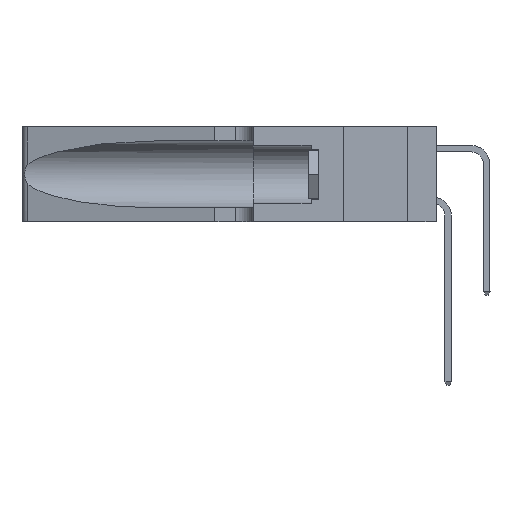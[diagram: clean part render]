
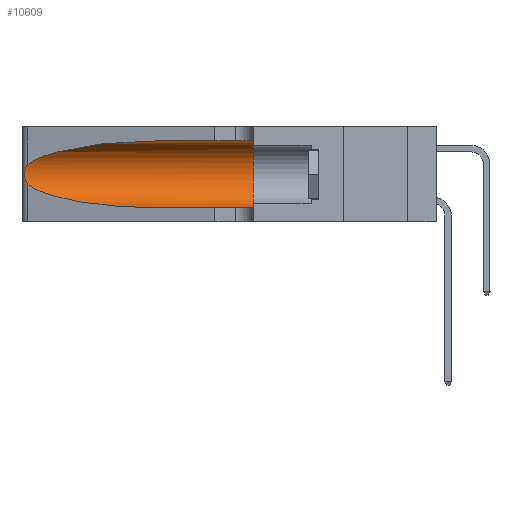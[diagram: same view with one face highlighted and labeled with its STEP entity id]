
A CAD part, left-side view. The second image highlights one B-rep face of the part: STEP entity #10609.
In plain terms, the highlighted cylindrical face has radius 3.308 mm (diameter 6.617 mm), a partial arc.
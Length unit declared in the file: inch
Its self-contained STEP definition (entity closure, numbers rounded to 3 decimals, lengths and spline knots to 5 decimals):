
#232 = CARTESIAN_POINT ( 'NONE',  ( 0.25789, 1.23486, 0.15765 ) ) ;
#282 = CARTESIAN_POINT ( 'NONE',  ( 0.25487, 1.22718, 0.22369 ) ) ;
#656 =( BOUNDED_CURVE ( )  B_SPLINE_CURVE ( 3, ( #3822, #26738, #10141, #18543 ),
 .UNSPECIFIED., .F., .F. ) 
 B_SPLINE_CURVE_WITH_KNOTS ( ( 4, 4 ),
 ( 3.44316, 4.71239 ),
 .UNSPECIFIED. ) 
 CURVE ( )  GEOMETRIC_REPRESENTATION_ITEM ( )  RATIONAL_B_SPLINE_CURVE ( ( 1., 0.87, 0.87, 1. ) ) 
 REPRESENTATION_ITEM ( '' )  );
#1777 = VERTEX_POINT ( 'NONE', #18138 ) ;
#2308 = CARTESIAN_POINT ( 'NONE',  ( 0.25487, 1.22718, 0.22369 ) ) ;
#2403 = CARTESIAN_POINT ( 'NONE',  ( 0.25555, 1.22993, 0.14849 ) ) ;
#2405 = ORIENTED_EDGE ( 'NONE', *, *, #3024, .F. ) ;
#3024 = EDGE_CURVE ( 'NONE', #24412, #22447, #14828, .T. ) ;
#3822 = CARTESIAN_POINT ( 'NONE',  ( 0.25487, 1.22718, 0.14631 ) ) ;
#3905 = EDGE_CURVE ( 'NONE', #4734, #1777, #20931, .T. ) ;
#4068 = EDGE_CURVE ( 'NONE', #20470, #4734, #656, .T. ) ;
#4179 = DIRECTION ( 'NONE',  ( 0., 1., 0. ) ) ;
#4346 = EDGE_LOOP ( 'NONE', ( #7255, #17045, #26488, #23386, #22606, #2405 ) ) ;
#4648 = DIRECTION ( 'NONE',  ( 0., -1., 0. ) ) ;
#4654 = CARTESIAN_POINT ( 'NONE',  ( 0.1305, 0.72297, 0.31525 ) ) ;
#4734 = VERTEX_POINT ( 'NONE', #20768 ) ;
#6615 = CARTESIAN_POINT ( 'NONE',  ( 0.25787, 1.23484, 0.2124 ) ) ;
#7255 = ORIENTED_EDGE ( 'NONE', *, *, #11817, .T. ) ;
#7945 = EDGE_CURVE ( 'NONE', #22447, #1777, #19527, .T. ) ;
#8757 = CARTESIAN_POINT ( 'NONE',  ( 0.26018, 1.23835, 0.19895 ) ) ;
#9828 = VECTOR ( 'NONE', #16001, 39.37008 ) ;
#10141 = CARTESIAN_POINT ( 'NONE',  ( 0.18966, 0.96281, 0.05475 ) ) ;
#10609 = ADVANCED_FACE ( 'NONE', ( #25759 ), #14796, .F. ) ;
#10856 = CARTESIAN_POINT ( 'NONE',  ( 0.26075, 1.23896, 0.178 ) ) ;
#11059 = DIRECTION ( 'NONE',  ( 0., 0., -1. ) ) ;
#11817 = EDGE_CURVE ( 'NONE', #24412, #23357, #25556, .T. ) ;
#11956 = CARTESIAN_POINT ( 'NONE',  ( 0.25487, 1.22718, 0.22369 ) ) ;
#12934 = CARTESIAN_POINT ( 'NONE',  ( 0.18966, 0.96281, 0.31525 ) ) ;
#12967 = CARTESIAN_POINT ( 'NONE',  ( 0.25856, 1.23593, 0.16098 ) ) ;
#13262 = CARTESIAN_POINT ( 'NONE',  ( 0.1305, 0.35, 0.31525 ) ) ;
#13805 = DIRECTION ( 'NONE',  ( 0., -1., 0. ) ) ;
#13936 = B_SPLINE_CURVE_WITH_KNOTS ( 'NONE', 3,
 ( #2308, #15007, #19188, #6615, #21249, #8757, #23313, #10856, #25390, #12967, #232, #15100, #2403, #17183 ),
 .UNSPECIFIED., .F., .F.,
 ( 4, 2, 2, 2, 2, 2, 4 ),
 ( 0., 0.00027, 0.00053, 0.00107, 0.0016, 0.00187, 0.00214 ),
 .UNSPECIFIED. ) ;
#14796 = CYLINDRICAL_SURFACE ( 'NONE', #25042, 0.13025 ) ;
#14828 = LINE ( 'NONE', #18005, #25161 ) ;
#15007 = CARTESIAN_POINT ( 'NONE',  ( 0.25555, 1.22994, 0.2215 ) ) ;
#15100 = CARTESIAN_POINT ( 'NONE',  ( 0.25639, 1.23186, 0.15144 ) ) ;
#16001 = DIRECTION ( 'NONE',  ( 0., -1., 0. ) ) ;
#16808 = CARTESIAN_POINT ( 'NONE',  ( 0.1305, 0.35, 0.185 ) ) ;
#16852 = CARTESIAN_POINT ( 'NONE',  ( 0.25487, 1.22718, 0.14631 ) ) ;
#17045 = ORIENTED_EDGE ( 'NONE', *, *, #22992, .T. ) ;
#17183 = CARTESIAN_POINT ( 'NONE',  ( 0.25487, 1.22718, 0.14631 ) ) ;
#18005 = CARTESIAN_POINT ( 'NONE',  ( 0.1305, 1.61858, 0.31525 ) ) ;
#18138 = CARTESIAN_POINT ( 'NONE',  ( 0.1305, 0.35, 0.05475 ) ) ;
#18355 = AXIS2_PLACEMENT_3D ( 'NONE', #16808, #4179, #18892 ) ;
#18543 = CARTESIAN_POINT ( 'NONE',  ( 0.1305, 0.72297, 0.05475 ) ) ;
#18892 = DIRECTION ( 'NONE',  ( 0., 0., 1. ) ) ;
#19188 = CARTESIAN_POINT ( 'NONE',  ( 0.25639, 1.23184, 0.21858 ) ) ;
#19527 = CIRCLE ( 'NONE', #18355, 0.13025 ) ;
#20470 = VERTEX_POINT ( 'NONE', #16852 ) ;
#20768 = CARTESIAN_POINT ( 'NONE',  ( 0.1305, 0.72297, 0.05475 ) ) ;
#20931 = LINE ( 'NONE', #22038, #9828 ) ;
#21249 = CARTESIAN_POINT ( 'NONE',  ( 0.25854, 1.2359, 0.20912 ) ) ;
#21300 = CARTESIAN_POINT ( 'NONE',  ( 0.2373, 1.15595, 0.28018 ) ) ;
#22038 = CARTESIAN_POINT ( 'NONE',  ( 0.1305, 1.61858, 0.05475 ) ) ;
#22447 = VERTEX_POINT ( 'NONE', #13262 ) ;
#22606 = ORIENTED_EDGE ( 'NONE', *, *, #7945, .F. ) ;
#22992 = EDGE_CURVE ( 'NONE', #23357, #20470, #13936, .T. ) ;
#23313 = CARTESIAN_POINT ( 'NONE',  ( 0.26075, 1.23896, 0.19203 ) ) ;
#23357 = VERTEX_POINT ( 'NONE', #11956 ) ;
#23386 = ORIENTED_EDGE ( 'NONE', *, *, #3905, .T. ) ;
#23514 = CARTESIAN_POINT ( 'NONE',  ( 0.1305, 1.61858, 0.185 ) ) ;
#24412 = VERTEX_POINT ( 'NONE', #4654 ) ;
#25042 = AXIS2_PLACEMENT_3D ( 'NONE', #23514, #4648, #11059 ) ;
#25161 = VECTOR ( 'NONE', #13805, 39.37008 ) ;
#25390 = CARTESIAN_POINT ( 'NONE',  ( 0.26017, 1.23833, 0.17102 ) ) ;
#25449 = CARTESIAN_POINT ( 'NONE',  ( 0.1305, 0.72297, 0.31525 ) ) ;
#25556 =( BOUNDED_CURVE ( )  B_SPLINE_CURVE ( 3, ( #25449, #12934, #21300, #282 ),
 .UNSPECIFIED., .F., .F. ) 
 B_SPLINE_CURVE_WITH_KNOTS ( ( 4, 4 ),
 ( 1.5708, 2.84003 ),
 .UNSPECIFIED. ) 
 CURVE ( )  GEOMETRIC_REPRESENTATION_ITEM ( )  RATIONAL_B_SPLINE_CURVE ( ( 1., 0.87, 0.87, 1. ) ) 
 REPRESENTATION_ITEM ( '' )  );
#25759 = FACE_OUTER_BOUND ( 'NONE', #4346, .T. ) ;
#26488 = ORIENTED_EDGE ( 'NONE', *, *, #4068, .T. ) ;
#26738 = CARTESIAN_POINT ( 'NONE',  ( 0.2373, 1.15595, 0.08982 ) ) ;
